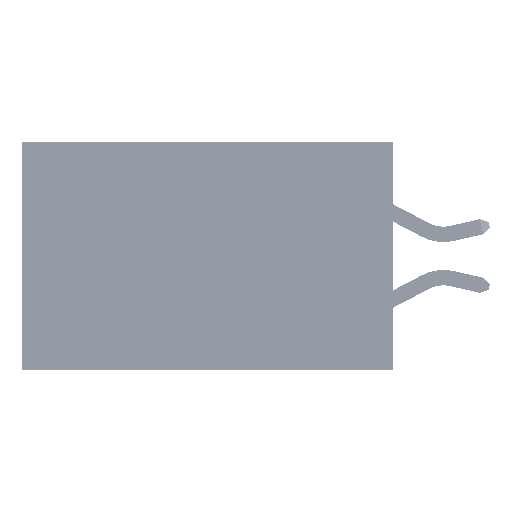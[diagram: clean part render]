
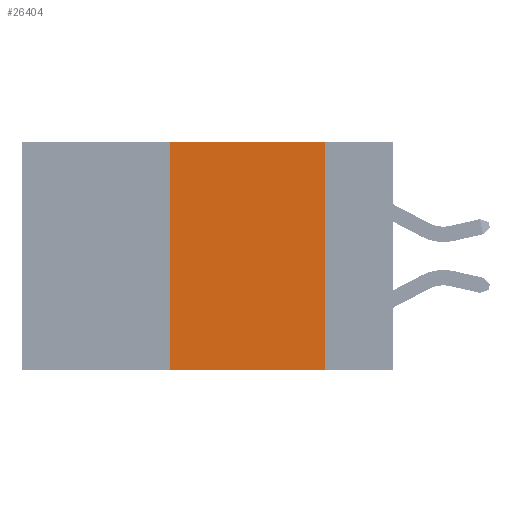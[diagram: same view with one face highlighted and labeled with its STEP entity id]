
A CAD part, left-side view. The second image highlights one B-rep face of the part: STEP entity #26404.
In plain terms, the highlighted planar face has unit normal (-1, 0, 0).
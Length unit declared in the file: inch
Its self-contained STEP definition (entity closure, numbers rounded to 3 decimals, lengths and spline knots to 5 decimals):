
#438 = EDGE_LOOP ( 'NONE', ( #27096, #21831, #36153, #6993 ) ) ;
#1592 = DIRECTION ( 'NONE',  ( 0., 0., -1. ) ) ;
#4012 = VECTOR ( 'NONE', #20712, 39.37008 ) ;
#4525 = LINE ( 'NONE', #41454, #34357 ) ;
#6509 = PLANE ( 'NONE',  #43970 ) ;
#6993 = ORIENTED_EDGE ( 'NONE', *, *, #29746, .T. ) ;
#7512 = CARTESIAN_POINT ( 'NONE',  ( 0., 0.36, -0.37 ) ) ;
#7557 = VERTEX_POINT ( 'NONE', #7512 ) ;
#12166 = EDGE_CURVE ( 'NONE', #7557, #30761, #4525, .T. ) ;
#12842 = CARTESIAN_POINT ( 'NONE',  ( 0., 0.36, 0. ) ) ;
#14417 = DIRECTION ( 'NONE',  ( 0., 0., -1. ) ) ;
#16548 = VERTEX_POINT ( 'NONE', #26046 ) ;
#16807 = CARTESIAN_POINT ( 'NONE',  ( 0., 0.6, 0. ) ) ;
#18433 = VECTOR ( 'NONE', #1592, 39.37008 ) ;
#20712 = DIRECTION ( 'NONE',  ( 0., -1., 0. ) ) ;
#21831 = ORIENTED_EDGE ( 'NONE', *, *, #30202, .F. ) ;
#22214 = DIRECTION ( 'NONE',  ( 0., 0., 1. ) ) ;
#24816 = VECTOR ( 'NONE', #37334, 39.37008 ) ;
#26046 = CARTESIAN_POINT ( 'NONE',  ( 0., 0.11, 0. ) ) ;
#26279 = EDGE_CURVE ( 'NONE', #16548, #32333, #39000, .T. ) ;
#26404 = ADVANCED_FACE ( 'NONE', ( #43199 ), #6509, .F. ) ;
#27096 = ORIENTED_EDGE ( 'NONE', *, *, #26279, .F. ) ;
#29746 = EDGE_CURVE ( 'NONE', #7557, #32333, #36321, .T. ) ;
#30202 = EDGE_CURVE ( 'NONE', #30761, #16548, #35069, .T. ) ;
#30761 = VERTEX_POINT ( 'NONE', #12842 ) ;
#32333 = VERTEX_POINT ( 'NONE', #36541 ) ;
#34357 = VECTOR ( 'NONE', #22214, 39.37008 ) ;
#35069 = LINE ( 'NONE', #16807, #4012 ) ;
#36153 = ORIENTED_EDGE ( 'NONE', *, *, #12166, .F. ) ;
#36321 = LINE ( 'NONE', #48773, #24816 ) ;
#36541 = CARTESIAN_POINT ( 'NONE',  ( 0., 0.11, -0.37 ) ) ;
#37334 = DIRECTION ( 'NONE',  ( 0., -1., 0. ) ) ;
#37631 = DIRECTION ( 'NONE',  ( 1., 0., 0. ) ) ;
#39000 = LINE ( 'NONE', #44349, #18433 ) ;
#41454 = CARTESIAN_POINT ( 'NONE',  ( 0., 0.36, 0. ) ) ;
#43199 = FACE_OUTER_BOUND ( 'NONE', #438, .T. ) ;
#43970 = AXIS2_PLACEMENT_3D ( 'NONE', #45186, #37631, #14417 ) ;
#44349 = CARTESIAN_POINT ( 'NONE',  ( 0., 0.11, 0. ) ) ;
#45186 = CARTESIAN_POINT ( 'NONE',  ( 0., 0.6, 0. ) ) ;
#48773 = CARTESIAN_POINT ( 'NONE',  ( 0., 0.6, -0.37 ) ) ;
